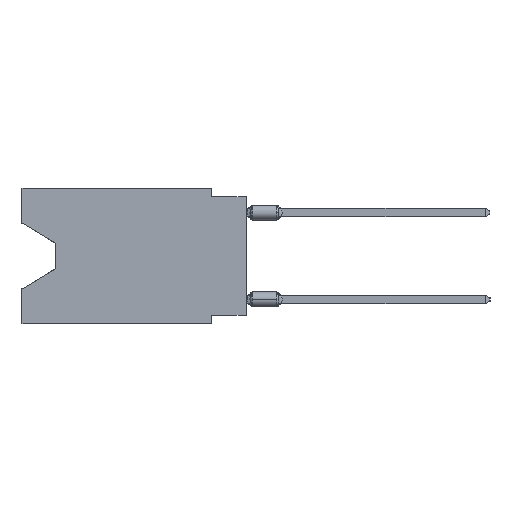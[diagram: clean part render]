
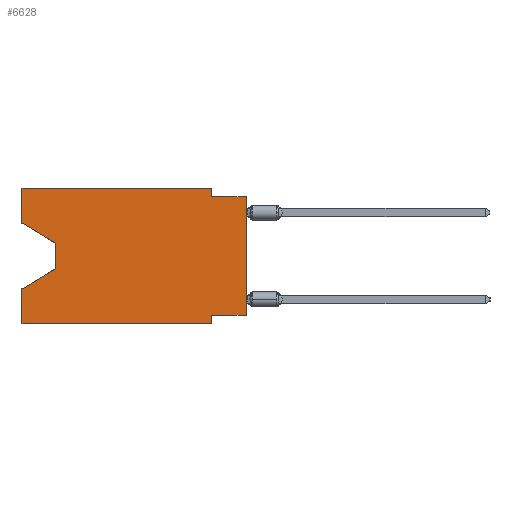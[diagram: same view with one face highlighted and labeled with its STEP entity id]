
A CAD part, left-side view. The second image highlights one B-rep face of the part: STEP entity #6628.
In plain terms, the highlighted planar face has unit normal (-1, 0, 0).
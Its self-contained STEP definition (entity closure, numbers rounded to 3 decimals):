
#529 = VERTEX_POINT ( 'NONE', #36716 ) ;
#1002 = ORIENTED_EDGE ( 'NONE', *, *, #28224, .T. ) ;
#1231 = CARTESIAN_POINT ( 'NONE',  ( 0., 16.383, -2.546 ) ) ;
#1465 = LINE ( 'NONE', #38691, #2000 ) ;
#2000 = VECTOR ( 'NONE', #11007, 1000. ) ;
#2761 = EDGE_CURVE ( 'NONE', #10809, #529, #14564, .T. ) ;
#3494 = VECTOR ( 'NONE', #28802, 1000. ) ;
#3660 = ORIENTED_EDGE ( 'NONE', *, *, #40951, .F. ) ;
#4117 = VECTOR ( 'NONE', #36450, 1000. ) ;
#4456 = VERTEX_POINT ( 'NONE', #15372 ) ;
#4701 = ORIENTED_EDGE ( 'NONE', *, *, #12126, .F. ) ;
#5281 = CARTESIAN_POINT ( 'NONE',  ( 0., 16.383, 0. ) ) ;
#6265 = VERTEX_POINT ( 'NONE', #42145 ) ;
#6628 = ADVANCED_FACE ( 'NONE', ( #22094 ), #35639, .F. ) ;
#6963 = VERTEX_POINT ( 'NONE', #34924 ) ;
#8240 = VERTEX_POINT ( 'NONE', #28510 ) ;
#8981 = LINE ( 'NONE', #12084, #11840 ) ;
#9319 = ORIENTED_EDGE ( 'NONE', *, *, #18710, .F. ) ;
#9506 = CARTESIAN_POINT ( 'NONE',  ( 0., 2.54, -9.906 ) ) ;
#10809 = VERTEX_POINT ( 'NONE', #1231 ) ;
#11007 = DIRECTION ( 'NONE',  ( 0., 1., 0. ) ) ;
#11121 = ORIENTED_EDGE ( 'NONE', *, *, #35387, .F. ) ;
#11828 = CARTESIAN_POINT ( 'NONE',  ( 0., 13.97, -4.013 ) ) ;
#11840 = VECTOR ( 'NONE', #25613, 1000. ) ;
#12006 = EDGE_CURVE ( 'NONE', #4456, #39247, #1465, .T. ) ;
#12084 = CARTESIAN_POINT ( 'NONE',  ( 0., 16.383, -2.546 ) ) ;
#12107 = VECTOR ( 'NONE', #24338, 1000. ) ;
#12126 = EDGE_CURVE ( 'NONE', #27388, #14812, #19556, .T. ) ;
#12628 = VECTOR ( 'NONE', #23772, 1000. ) ;
#14564 = LINE ( 'NONE', #31421, #12107 ) ;
#14812 = VERTEX_POINT ( 'NONE', #14951 ) ;
#14951 = CARTESIAN_POINT ( 'NONE',  ( 0., 16.383, -7.36 ) ) ;
#15372 = CARTESIAN_POINT ( 'NONE',  ( 0., 0., -9.271 ) ) ;
#15379 = ORIENTED_EDGE ( 'NONE', *, *, #33442, .F. ) ;
#15427 = DIRECTION ( 'NONE',  ( 1., 0., 0. ) ) ;
#16192 = LINE ( 'NONE', #16839, #41003 ) ;
#16567 = DIRECTION ( 'NONE',  ( 0., 0., -1. ) ) ;
#16839 = CARTESIAN_POINT ( 'NONE',  ( 0., 16.383, -9.906 ) ) ;
#16981 = LINE ( 'NONE', #9506, #29716 ) ;
#17143 = DIRECTION ( 'NONE',  ( 0., -1., 0. ) ) ;
#17757 = DIRECTION ( 'NONE',  ( 0., 0., 1. ) ) ;
#18337 = CARTESIAN_POINT ( 'NONE',  ( 0., 16.383, -9.906 ) ) ;
#18642 = ORIENTED_EDGE ( 'NONE', *, *, #33593, .T. ) ;
#18710 = EDGE_CURVE ( 'NONE', #8240, #28865, #25462, .T. ) ;
#19556 = LINE ( 'NONE', #32442, #4117 ) ;
#19688 = VECTOR ( 'NONE', #17143, 1000. ) ;
#19974 = ORIENTED_EDGE ( 'NONE', *, *, #2761, .F. ) ;
#20493 = VERTEX_POINT ( 'NONE', #22285 ) ;
#21115 = CARTESIAN_POINT ( 'NONE',  ( 0., 13.97, -4.013 ) ) ;
#21221 = VECTOR ( 'NONE', #25352, 1000. ) ;
#22094 = FACE_OUTER_BOUND ( 'NONE', #29813, .T. ) ;
#22246 = ORIENTED_EDGE ( 'NONE', *, *, #36287, .T. ) ;
#22285 = CARTESIAN_POINT ( 'NONE',  ( 0., 2.54, -9.906 ) ) ;
#22952 = LINE ( 'NONE', #36492, #3494 ) ;
#23216 = CARTESIAN_POINT ( 'NONE',  ( 0., 2.54, -0.635 ) ) ;
#23538 = ORIENTED_EDGE ( 'NONE', *, *, #12006, .F. ) ;
#23772 = DIRECTION ( 'NONE',  ( 0., 0.855, -0.519 ) ) ;
#24338 = DIRECTION ( 'NONE',  ( 0., 0., 1. ) ) ;
#25009 = DIRECTION ( 'NONE',  ( 0., 0., -1. ) ) ;
#25352 = DIRECTION ( 'NONE',  ( 0., 0., -1. ) ) ;
#25462 = LINE ( 'NONE', #38774, #30003 ) ;
#25613 = DIRECTION ( 'NONE',  ( 0., -0.855, -0.519 ) ) ;
#25803 = LINE ( 'NONE', #39324, #12628 ) ;
#26380 = VERTEX_POINT ( 'NONE', #21115 ) ;
#26644 = DIRECTION ( 'NONE',  ( 0., -1., 0. ) ) ;
#27388 = VERTEX_POINT ( 'NONE', #18337 ) ;
#28135 = CARTESIAN_POINT ( 'NONE',  ( 0., 2.54, -9.271 ) ) ;
#28224 = EDGE_CURVE ( 'NONE', #26380, #6963, #28238, .T. ) ;
#28238 = LINE ( 'NONE', #11828, #21221 ) ;
#28510 = CARTESIAN_POINT ( 'NONE',  ( 0., 2.54, 0. ) ) ;
#28802 = DIRECTION ( 'NONE',  ( 0., -1., 0. ) ) ;
#28865 = VERTEX_POINT ( 'NONE', #23216 ) ;
#29716 = VECTOR ( 'NONE', #16567, 1000. ) ;
#29763 = LINE ( 'NONE', #41521, #37591 ) ;
#29813 = EDGE_LOOP ( 'NONE', ( #35768, #1002, #31871, #4701, #18642, #11121, #23538, #22246, #3660, #9319, #15379, #19974 ) ) ;
#30003 = VECTOR ( 'NONE', #35674, 1000. ) ;
#31421 = CARTESIAN_POINT ( 'NONE',  ( 0., 16.383, 0. ) ) ;
#31871 = ORIENTED_EDGE ( 'NONE', *, *, #40219, .T. ) ;
#31985 = EDGE_CURVE ( 'NONE', #10809, #26380, #8981, .T. ) ;
#32442 = CARTESIAN_POINT ( 'NONE',  ( 0., 16.383, 0. ) ) ;
#33442 = EDGE_CURVE ( 'NONE', #529, #8240, #41559, .T. ) ;
#33593 = EDGE_CURVE ( 'NONE', #27388, #20493, #16192, .T. ) ;
#34924 = CARTESIAN_POINT ( 'NONE',  ( 0., 13.97, -5.893 ) ) ;
#35387 = EDGE_CURVE ( 'NONE', #39247, #20493, #16981, .T. ) ;
#35639 = PLANE ( 'NONE',  #42068 ) ;
#35674 = DIRECTION ( 'NONE',  ( 0., 0., -1. ) ) ;
#35768 = ORIENTED_EDGE ( 'NONE', *, *, #31985, .T. ) ;
#36287 = EDGE_CURVE ( 'NONE', #4456, #6265, #29763, .T. ) ;
#36450 = DIRECTION ( 'NONE',  ( 0., 0., 1. ) ) ;
#36492 = CARTESIAN_POINT ( 'NONE',  ( 0., 0., -0.635 ) ) ;
#36716 = CARTESIAN_POINT ( 'NONE',  ( 0., 16.383, 0. ) ) ;
#37591 = VECTOR ( 'NONE', #17757, 1000. ) ;
#37803 = CARTESIAN_POINT ( 'NONE',  ( 0., 16.383, 0. ) ) ;
#38691 = CARTESIAN_POINT ( 'NONE',  ( 0., 0., -9.271 ) ) ;
#38774 = CARTESIAN_POINT ( 'NONE',  ( 0., 2.54, 0. ) ) ;
#39247 = VERTEX_POINT ( 'NONE', #28135 ) ;
#39324 = CARTESIAN_POINT ( 'NONE',  ( 0., 13.97, -5.893 ) ) ;
#40219 = EDGE_CURVE ( 'NONE', #6963, #14812, #25803, .T. ) ;
#40951 = EDGE_CURVE ( 'NONE', #28865, #6265, #22952, .T. ) ;
#41003 = VECTOR ( 'NONE', #26644, 1000. ) ;
#41521 = CARTESIAN_POINT ( 'NONE',  ( 0., 0., 0. ) ) ;
#41559 = LINE ( 'NONE', #37803, #19688 ) ;
#42068 = AXIS2_PLACEMENT_3D ( 'NONE', #5281, #15427, #25009 ) ;
#42145 = CARTESIAN_POINT ( 'NONE',  ( 0., 0., -0.635 ) ) ;
